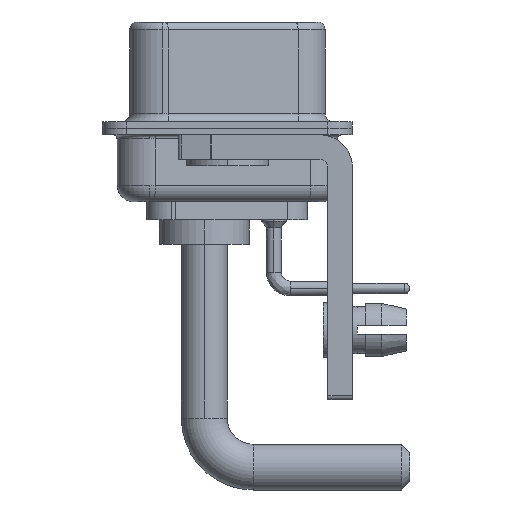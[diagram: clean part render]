
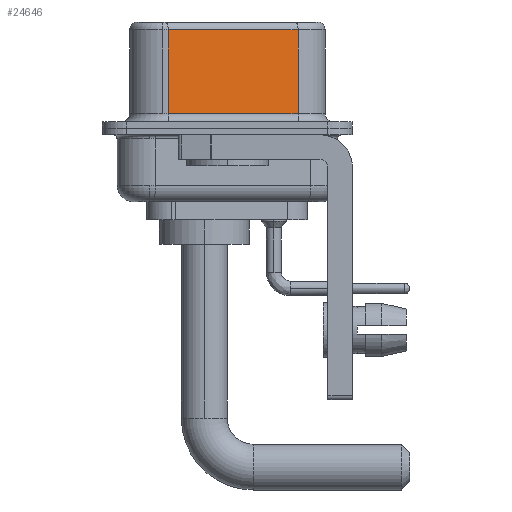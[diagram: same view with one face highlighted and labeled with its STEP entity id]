
A CAD part, left-side view. The second image highlights one B-rep face of the part: STEP entity #24646.
In plain terms, the highlighted planar face has unit normal (-0.985, -0.174, 0).
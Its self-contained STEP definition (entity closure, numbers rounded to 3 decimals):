
#222 = CARTESIAN_POINT ( 'NONE',  ( 5.132, -4.322, 0.9 ) ) ;
#985 = ORIENTED_EDGE ( 'NONE', *, *, #5511, .T. ) ;
#1076 = AXIS2_PLACEMENT_3D ( 'NONE', #21302, #1107, #9205 ) ;
#1107 = DIRECTION ( 'NONE',  ( 0.985, 0.174, 0. ) ) ;
#1408 = LINE ( 'NONE', #7534, #18517 ) ;
#2326 = CARTESIAN_POINT ( 'NONE',  ( 5.132, -4.322, 6.52 ) ) ;
#2598 = ORIENTED_EDGE ( 'NONE', *, *, #15228, .T. ) ;
#2963 = CARTESIAN_POINT ( 'NONE',  ( 5.132, -4.322, 6.02 ) ) ;
#3120 = LINE ( 'NONE', #23045, #18859 ) ;
#5285 = VERTEX_POINT ( 'NONE', #222 ) ;
#5511 = EDGE_CURVE ( 'NONE', #9075, #22262, #9392, .T. ) ;
#5864 = CARTESIAN_POINT ( 'NONE',  ( 3.73, 3.628, 0.9 ) ) ;
#6777 = VECTOR ( 'NONE', #11121, 1000. ) ;
#7534 = CARTESIAN_POINT ( 'NONE',  ( 5.132, -4.322, 6.02 ) ) ;
#9075 = VERTEX_POINT ( 'NONE', #26272 ) ;
#9205 = DIRECTION ( 'NONE',  ( -0.174, 0.985, 0. ) ) ;
#9392 = LINE ( 'NONE', #13632, #6777 ) ;
#9412 = ORIENTED_EDGE ( 'NONE', *, *, #12464, .F. ) ;
#11121 = DIRECTION ( 'NONE',  ( 0., 0., -1. ) ) ;
#12464 = EDGE_CURVE ( 'NONE', #13022, #5285, #24515, .T. ) ;
#13022 = VERTEX_POINT ( 'NONE', #2963 ) ;
#13185 = PLANE ( 'NONE',  #1076 ) ;
#13632 = CARTESIAN_POINT ( 'NONE',  ( 3.73, 3.628, 6.52 ) ) ;
#15228 = EDGE_CURVE ( 'NONE', #22262, #5285, #3120, .T. ) ;
#15618 = DIRECTION ( 'NONE',  ( -0.174, 0.985, 0. ) ) ;
#18143 = DIRECTION ( 'NONE',  ( 0., 0., -1. ) ) ;
#18517 = VECTOR ( 'NONE', #15618, 1000. ) ;
#18859 = VECTOR ( 'NONE', #25040, 1000. ) ;
#19589 = EDGE_CURVE ( 'NONE', #13022, #9075, #1408, .T. ) ;
#19635 = VECTOR ( 'NONE', #18143, 1000. ) ;
#19956 = ORIENTED_EDGE ( 'NONE', *, *, #19589, .T. ) ;
#21302 = CARTESIAN_POINT ( 'NONE',  ( 5.132, -4.322, 6.52 ) ) ;
#22262 = VERTEX_POINT ( 'NONE', #5864 ) ;
#23045 = CARTESIAN_POINT ( 'NONE',  ( 5.132, -4.322, 0.9 ) ) ;
#23311 = FACE_OUTER_BOUND ( 'NONE', #24185, .T. ) ;
#24185 = EDGE_LOOP ( 'NONE', ( #9412, #19956, #985, #2598 ) ) ;
#24515 = LINE ( 'NONE', #2326, #19635 ) ;
#24646 = ADVANCED_FACE ( 'NONE', ( #23311 ), #13185, .F. ) ;
#25040 = DIRECTION ( 'NONE',  ( 0.174, -0.985, 0. ) ) ;
#26272 = CARTESIAN_POINT ( 'NONE',  ( 3.73, 3.628, 6.02 ) ) ;
